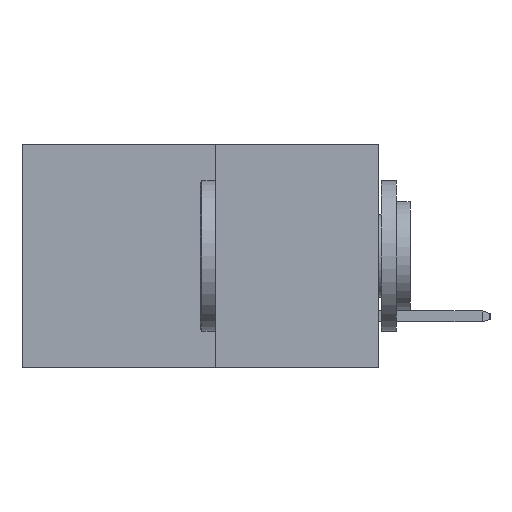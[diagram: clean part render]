
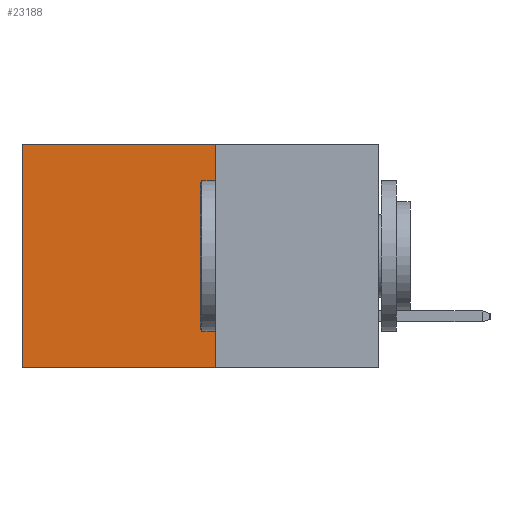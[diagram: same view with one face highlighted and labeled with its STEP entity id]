
A CAD part, left-side view. The second image highlights one B-rep face of the part: STEP entity #23188.
In plain terms, the highlighted planar face has unit normal (-1, 0, 0).
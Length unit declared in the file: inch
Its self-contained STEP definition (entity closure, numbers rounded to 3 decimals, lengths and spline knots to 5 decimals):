
#1171 = VECTOR ( 'NONE', #4189, 39.37008 ) ;
#2939 = CARTESIAN_POINT ( 'NONE',  ( 0.277, 0.27, -0.37 ) ) ;
#3674 = LINE ( 'NONE', #5489, #28409 ) ;
#4028 = ORIENTED_EDGE ( 'NONE', *, *, #12715, .F. ) ;
#4189 = DIRECTION ( 'NONE',  ( 0., 1., 0. ) ) ;
#4743 = VERTEX_POINT ( 'NONE', #29555 ) ;
#4943 = EDGE_CURVE ( 'NONE', #4743, #16980, #21422, .T. ) ;
#5293 = DIRECTION ( 'NONE',  ( 0., 0., -1. ) ) ;
#5489 = CARTESIAN_POINT ( 'NONE',  ( 0.277, 0.27, -0.37 ) ) ;
#7374 = LINE ( 'NONE', #27278, #1171 ) ;
#11598 = EDGE_CURVE ( 'NONE', #12380, #12265, #18612, .T. ) ;
#12265 = VERTEX_POINT ( 'NONE', #27185 ) ;
#12380 = VERTEX_POINT ( 'NONE', #22971 ) ;
#12463 = CARTESIAN_POINT ( 'NONE',  ( 0.277, 0.59, -0.37 ) ) ;
#12715 = EDGE_CURVE ( 'NONE', #12265, #16980, #3674, .T. ) ;
#12742 = CARTESIAN_POINT ( 'NONE',  ( 0.277, 0.27, -0.37 ) ) ;
#14640 = EDGE_LOOP ( 'NONE', ( #25620, #4028, #16807, #19894 ) ) ;
#14690 = DIRECTION ( 'NONE',  ( 0., 1., 0. ) ) ;
#15041 = DIRECTION ( 'NONE',  ( 0., 0., -1. ) ) ;
#16807 = ORIENTED_EDGE ( 'NONE', *, *, #11598, .F. ) ;
#16980 = VERTEX_POINT ( 'NONE', #12463 ) ;
#17929 = CARTESIAN_POINT ( 'NONE',  ( 0.277, 0.59, -0.37 ) ) ;
#18612 = LINE ( 'NONE', #12742, #25601 ) ;
#19153 = DIRECTION ( 'NONE',  ( 1., 0., 0. ) ) ;
#19894 = ORIENTED_EDGE ( 'NONE', *, *, #24799, .T. ) ;
#21422 = LINE ( 'NONE', #17929, #27641 ) ;
#22361 = FACE_OUTER_BOUND ( 'NONE', #14640, .T. ) ;
#22514 = AXIS2_PLACEMENT_3D ( 'NONE', #2939, #19153, #5293 ) ;
#22637 = DIRECTION ( 'NONE',  ( 0., 0., -1. ) ) ;
#22971 = CARTESIAN_POINT ( 'NONE',  ( 0.277, 0.27, 0. ) ) ;
#23188 = ADVANCED_FACE ( 'NONE', ( #22361 ), #28454, .F. ) ;
#24799 = EDGE_CURVE ( 'NONE', #12380, #4743, #7374, .T. ) ;
#25601 = VECTOR ( 'NONE', #15041, 39.37008 ) ;
#25620 = ORIENTED_EDGE ( 'NONE', *, *, #4943, .T. ) ;
#27185 = CARTESIAN_POINT ( 'NONE',  ( 0.277, 0.27, -0.37 ) ) ;
#27278 = CARTESIAN_POINT ( 'NONE',  ( 0.277, 0.27, 0. ) ) ;
#27641 = VECTOR ( 'NONE', #22637, 39.37008 ) ;
#28409 = VECTOR ( 'NONE', #14690, 39.37008 ) ;
#28454 = PLANE ( 'NONE',  #22514 ) ;
#29555 = CARTESIAN_POINT ( 'NONE',  ( 0.277, 0.59, 0. ) ) ;
